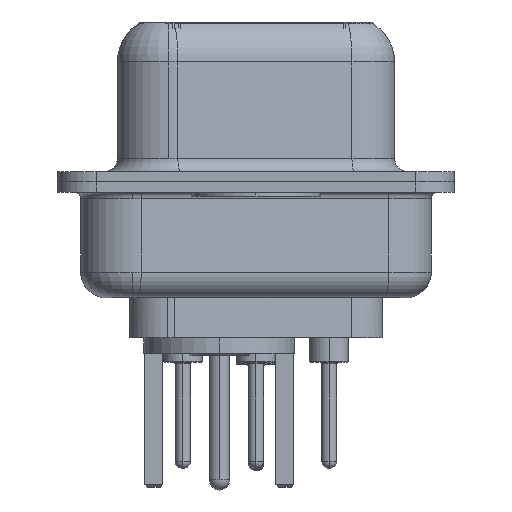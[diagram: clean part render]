
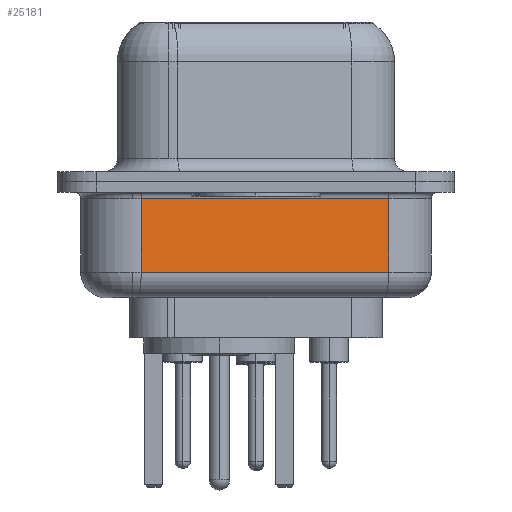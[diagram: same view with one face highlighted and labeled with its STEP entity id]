
A CAD part, left-side view. The second image highlights one B-rep face of the part: STEP entity #25181.
In plain terms, the highlighted planar face has unit normal (-0.985, -0.174, 0).
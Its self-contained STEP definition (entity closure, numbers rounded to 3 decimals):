
#97 = ORIENTED_EDGE ( 'NONE', *, *, #2040, .F. ) ;
#975 = CARTESIAN_POINT ( 'NONE',  ( 2.93, 4.453, -3.5 ) ) ;
#1144 = CARTESIAN_POINT ( 'NONE',  ( 2.93, 4.453, -0.65 ) ) ;
#1729 = CARTESIAN_POINT ( 'NONE',  ( 4.623, -5.147, -0.65 ) ) ;
#2035 = LINE ( 'NONE', #975, #21903 ) ;
#2040 = EDGE_CURVE ( 'NONE', #22185, #7616, #13175, .T. ) ;
#6477 = DIRECTION ( 'NONE',  ( -0.174, 0.985, 0. ) ) ;
#7616 = VERTEX_POINT ( 'NONE', #19193 ) ;
#7835 = CARTESIAN_POINT ( 'NONE',  ( 4.623, -5.147, -4.5 ) ) ;
#9045 = LINE ( 'NONE', #1144, #19597 ) ;
#13126 = CARTESIAN_POINT ( 'NONE',  ( 2.93, 4.453, -4.5 ) ) ;
#13175 = LINE ( 'NONE', #13126, #14800 ) ;
#13432 = PLANE ( 'NONE',  #25949 ) ;
#14007 = ORIENTED_EDGE ( 'NONE', *, *, #27560, .T. ) ;
#14800 = VECTOR ( 'NONE', #15747, 1000. ) ;
#15593 = FACE_OUTER_BOUND ( 'NONE', #31415, .T. ) ;
#15747 = DIRECTION ( 'NONE',  ( 0., 0., 1. ) ) ;
#19193 = CARTESIAN_POINT ( 'NONE',  ( 2.93, 4.453, -0.65 ) ) ;
#19597 = VECTOR ( 'NONE', #6477, 1000. ) ;
#20379 = CARTESIAN_POINT ( 'NONE',  ( 2.93, 4.453, -3.5 ) ) ;
#21763 = EDGE_CURVE ( 'NONE', #22185, #24864, #2035, .T. ) ;
#21903 = VECTOR ( 'NONE', #32343, 1000. ) ;
#21926 = CARTESIAN_POINT ( 'NONE',  ( 4.623, -5.147, -3.5 ) ) ;
#22185 = VERTEX_POINT ( 'NONE', #20379 ) ;
#24160 = LINE ( 'NONE', #7835, #29858 ) ;
#24864 = VERTEX_POINT ( 'NONE', #21926 ) ;
#25181 = ADVANCED_FACE ( 'NONE', ( #15593 ), #13432, .F. ) ;
#25927 = DIRECTION ( 'NONE',  ( 0., 0., 1. ) ) ;
#25949 = AXIS2_PLACEMENT_3D ( 'NONE', #28899, #31204, #26404 ) ;
#25987 = EDGE_CURVE ( 'NONE', #27307, #7616, #9045, .T. ) ;
#26404 = DIRECTION ( 'NONE',  ( -0.174, 0.985, 0. ) ) ;
#26659 = ORIENTED_EDGE ( 'NONE', *, *, #25987, .T. ) ;
#27307 = VERTEX_POINT ( 'NONE', #1729 ) ;
#27560 = EDGE_CURVE ( 'NONE', #24864, #27307, #24160, .T. ) ;
#28899 = CARTESIAN_POINT ( 'NONE',  ( 2.93, 4.453, -4.5 ) ) ;
#29858 = VECTOR ( 'NONE', #25927, 1000. ) ;
#29953 = ORIENTED_EDGE ( 'NONE', *, *, #21763, .T. ) ;
#31204 = DIRECTION ( 'NONE',  ( 0.985, 0.174, 0. ) ) ;
#31415 = EDGE_LOOP ( 'NONE', ( #97, #29953, #14007, #26659 ) ) ;
#32343 = DIRECTION ( 'NONE',  ( 0.174, -0.985, 0. ) ) ;
